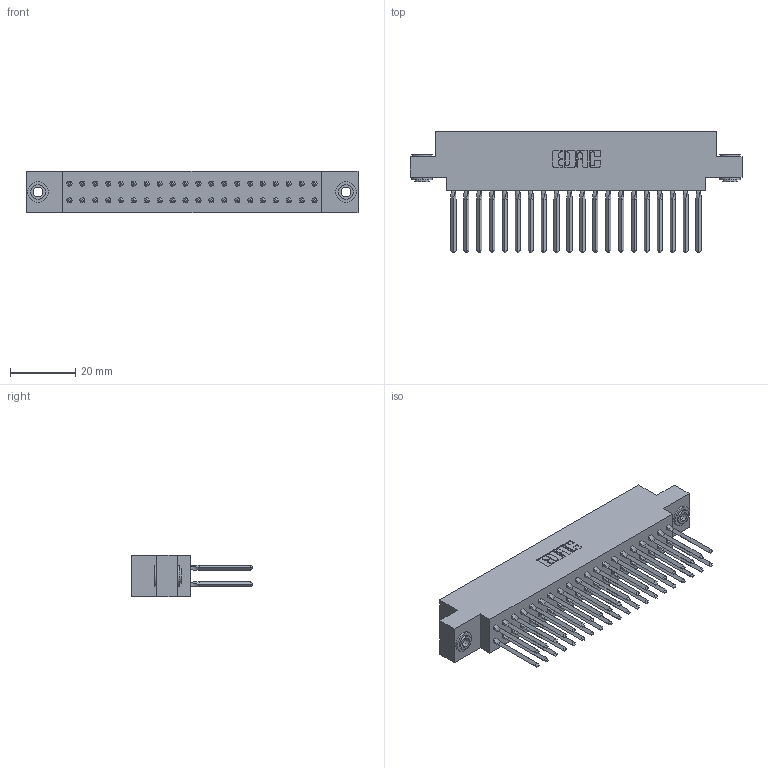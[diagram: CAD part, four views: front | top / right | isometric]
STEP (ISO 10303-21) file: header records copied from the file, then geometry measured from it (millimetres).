
FILE_DESCRIPTION (( 'STEP AP203' ), '1' );
FILE_NAME ('317-040-540-803.STEP', '2020-02-28T00:27:11', ( '' ), ( '' ), 'SwSTEP 2.0', 'SolidWorks 2016', '' );
FILE_SCHEMA (( 'CONFIG_CONTROL_DESIGN' ));
Length unit declared in the file: inch
Products named in the file (4): 345-250-002_345-250-002-102; 317-290-001_540; 317 Part_.156 Dia - TH; 317-040-540-803
Assembly tree (43 placements, depth 2):
  317-040-540-803
    317 Part_.156 Dia - TH
    317-290-001_540  x40
    345-250-002_345-250-002-102  x2
Bounding box: 101.96 x 37.34 x 12.7 mm (x, y, z)
Volume: 16386.9 mm3; surface area: 23813.7 mm2
Topology: 43 solids, 43 shells, 3700 faces, 10231 edges, 6590 vertices
Faces by surface type: plane 2988, cylinder 544, bspline 160, cone 8
Entity records: 32629 total; most frequent: CARTESIAN_POINT 6074, ORIENTED_EDGE 5566, DIRECTION 4687, EDGE_CURVE 2783, LINE 2503, VECTOR 2503, VERTEX_POINT 1847, AXIS2_PLACEMENT_3D 1092
